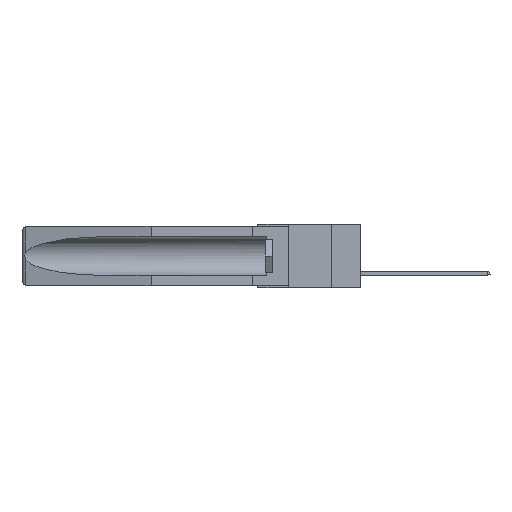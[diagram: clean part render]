
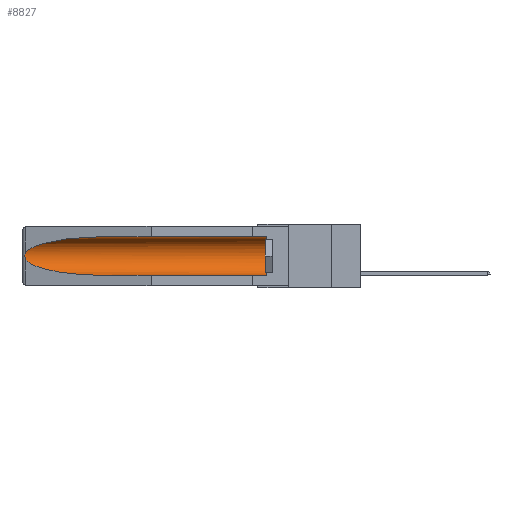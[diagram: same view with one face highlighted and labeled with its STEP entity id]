
A CAD part, left-side view. The second image highlights one B-rep face of the part: STEP entity #8827.
In plain terms, the highlighted cylindrical face has radius 2.857 mm (diameter 5.715 mm), a partial arc.
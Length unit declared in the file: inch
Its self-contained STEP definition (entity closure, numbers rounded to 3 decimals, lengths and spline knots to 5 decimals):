
#1058 = CARTESIAN_POINT ( 'NONE',  ( 0.21114, 1.30732, -0.059 ) ) ;
#1381 = CARTESIAN_POINT ( 'NONE',  ( 0.26597, 1.52961, -0.15275 ) ) ;
#2567 = EDGE_CURVE ( 'NONE', #7569, #7550, #28097, .T. ) ;
#3608 = CARTESIAN_POINT ( 'NONE',  ( 0.21114, 1.30732, -0.284 ) ) ;
#4143 = CARTESIAN_POINT ( 'NONE',  ( 0.155, 1.07973, -0.284 ) ) ;
#4687 = ORIENTED_EDGE ( 'NONE', *, *, #26482, .T. ) ;
#4973 = DIRECTION ( 'NONE',  ( 0., 0., 1. ) ) ;
#6035 = CARTESIAN_POINT ( 'NONE',  ( 0.26654, 1.53092, -0.15636 ) ) ;
#6379 = EDGE_CURVE ( 'NONE', #23837, #25212, #24492, .T. ) ;
#6479 = VECTOR ( 'NONE', #26241, 39.37008 ) ;
#6564 = CARTESIAN_POINT ( 'NONE',  ( 0.155, 0.126, -0.1715 ) ) ;
#7550 = VERTEX_POINT ( 'NONE', #22206 ) ;
#7569 = VERTEX_POINT ( 'NONE', #17108 ) ;
#7634 = ORIENTED_EDGE ( 'NONE', *, *, #6379, .F. ) ;
#8442 = CARTESIAN_POINT ( 'NONE',  ( 0.2673, 1.5327, -0.16383 ) ) ;
#8625 = CARTESIAN_POINT ( 'NONE',  ( 0.155, 0.126, -0.284 ) ) ;
#8755 = CARTESIAN_POINT ( 'NONE',  ( 0.155, 1.07973, -0.284 ) ) ;
#8827 = ADVANCED_FACE ( 'NONE', ( #15938 ), #14082, .F. ) ;
#9078 = CARTESIAN_POINT ( 'NONE',  ( 0.155, -0.30754, -0.059 ) ) ;
#9116 = AXIS2_PLACEMENT_3D ( 'NONE', #12078, #21536, #4973 ) ;
#9620 = VERTEX_POINT ( 'NONE', #16641 ) ;
#10300 = EDGE_CURVE ( 'NONE', #21762, #9620, #12823, .T. ) ;
#11055 = DIRECTION ( 'NONE',  ( 0., 0., 1. ) ) ;
#11269 = CARTESIAN_POINT ( 'NONE',  ( 0.26537, 1.52718, -0.14972 ) ) ;
#11272 = CARTESIAN_POINT ( 'NONE',  ( 0.26537, 1.52718, -0.19328 ) ) ;
#12078 = CARTESIAN_POINT ( 'NONE',  ( 0.155, -0.30754, -0.1715 ) ) ;
#12635 = CARTESIAN_POINT ( 'NONE',  ( 0.25451, 1.48313, -0.09465 ) ) ;
#12823 = LINE ( 'NONE', #9078, #6479 ) ;
#13181 =( BOUNDED_CURVE ( )  B_SPLINE_CURVE ( 3, ( #11272, #27703, #3608, #8755 ),
 .UNSPECIFIED., .F., .F. ) 
 B_SPLINE_CURVE_WITH_KNOTS ( ( 4, 4 ),
 ( 0.1948, 1.5708 ),
 .UNSPECIFIED. ) 
 CURVE ( )  GEOMETRIC_REPRESENTATION_ITEM ( )  RATIONAL_B_SPLINE_CURVE ( ( 1., 0.848, 0.848, 1. ) ) 
 REPRESENTATION_ITEM ( '' )  );
#13237 = CARTESIAN_POINT ( 'NONE',  ( 0.26597, 1.5296, -0.19026 ) ) ;
#13543 = DIRECTION ( 'NONE',  ( 0., -1., 0. ) ) ;
#14082 = CYLINDRICAL_SURFACE ( 'NONE', #9116, 0.1125 ) ;
#14152 = DIRECTION ( 'NONE',  ( 0., 1., 0. ) ) ;
#15310 = CARTESIAN_POINT ( 'NONE',  ( 0.155, 1.07973, -0.059 ) ) ;
#15515 = CARTESIAN_POINT ( 'NONE',  ( 0.26655, 1.53094, -0.18657 ) ) ;
#15938 = FACE_OUTER_BOUND ( 'NONE', #26857, .T. ) ;
#16641 = CARTESIAN_POINT ( 'NONE',  ( 0.155, 1.07973, -0.059 ) ) ;
#17108 = CARTESIAN_POINT ( 'NONE',  ( 0.26537, 1.52718, -0.14972 ) ) ;
#17974 = CARTESIAN_POINT ( 'NONE',  ( 0.155, 0.126, -0.059 ) ) ;
#19864 = EDGE_CURVE ( 'NONE', #7550, #25212, #13181, .T. ) ;
#21027 = CARTESIAN_POINT ( 'NONE',  ( 0.155, -0.30754, -0.284 ) ) ;
#21071 = VECTOR ( 'NONE', #14152, 39.37008 ) ;
#21536 = DIRECTION ( 'NONE',  ( 0., 1., 0. ) ) ;
#21762 = VERTEX_POINT ( 'NONE', #17974 ) ;
#22069 =( BOUNDED_CURVE ( )  B_SPLINE_CURVE ( 3, ( #15310, #1058, #12635, #29588 ),
 .UNSPECIFIED., .F., .F. ) 
 B_SPLINE_CURVE_WITH_KNOTS ( ( 4, 4 ),
 ( 4.71239, 6.08839 ),
 .UNSPECIFIED. ) 
 CURVE ( )  GEOMETRIC_REPRESENTATION_ITEM ( )  RATIONAL_B_SPLINE_CURVE ( ( 1., 0.848, 0.848, 1. ) ) 
 REPRESENTATION_ITEM ( '' )  );
#22206 = CARTESIAN_POINT ( 'NONE',  ( 0.26537, 1.52718, -0.19328 ) ) ;
#22503 = ORIENTED_EDGE ( 'NONE', *, *, #19864, .T. ) ;
#23251 = CARTESIAN_POINT ( 'NONE',  ( 0.2675, 1.53308, -0.16763 ) ) ;
#23837 = VERTEX_POINT ( 'NONE', #8625 ) ;
#24492 = LINE ( 'NONE', #21027, #21071 ) ;
#25212 = VERTEX_POINT ( 'NONE', #4143 ) ;
#25284 = CARTESIAN_POINT ( 'NONE',  ( 0.26537, 1.52718, -0.19328 ) ) ;
#26241 = DIRECTION ( 'NONE',  ( 0., 1., 0. ) ) ;
#26482 = EDGE_CURVE ( 'NONE', #23837, #21762, #26773, .T. ) ;
#26596 = ORIENTED_EDGE ( 'NONE', *, *, #2567, .T. ) ;
#26773 = CIRCLE ( 'NONE', #29479, 0.1125 ) ;
#26857 = EDGE_LOOP ( 'NONE', ( #30092, #26596, #22503, #7634, #4687, #29542 ) ) ;
#27703 = CARTESIAN_POINT ( 'NONE',  ( 0.25451, 1.48313, -0.24835 ) ) ;
#28097 = B_SPLINE_CURVE_WITH_KNOTS ( 'NONE', 3,
 ( #11269, #1381, #6035, #8442, #23251, #28124, #29989, #15515, #13237, #25284 ),
 .UNSPECIFIED., .F., .F.,
 ( 4, 2, 2, 2, 4 ),
 ( 0., 0.00029, 0.00058, 0.00087, 0.00117 ),
 .UNSPECIFIED. ) ;
#28124 = CARTESIAN_POINT ( 'NONE',  ( 0.2675, 1.53308, -0.17534 ) ) ;
#29127 = EDGE_CURVE ( 'NONE', #9620, #7569, #22069, .T. ) ;
#29479 = AXIS2_PLACEMENT_3D ( 'NONE', #6564, #13543, #11055 ) ;
#29542 = ORIENTED_EDGE ( 'NONE', *, *, #10300, .T. ) ;
#29588 = CARTESIAN_POINT ( 'NONE',  ( 0.26537, 1.52718, -0.14972 ) ) ;
#29989 = CARTESIAN_POINT ( 'NONE',  ( 0.2673, 1.53269, -0.17917 ) ) ;
#30092 = ORIENTED_EDGE ( 'NONE', *, *, #29127, .T. ) ;
